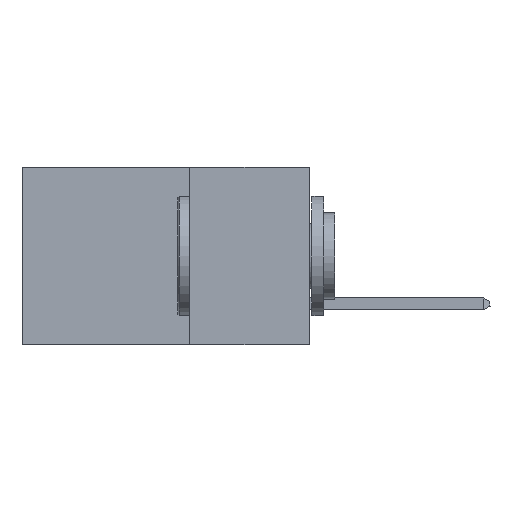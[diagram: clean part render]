
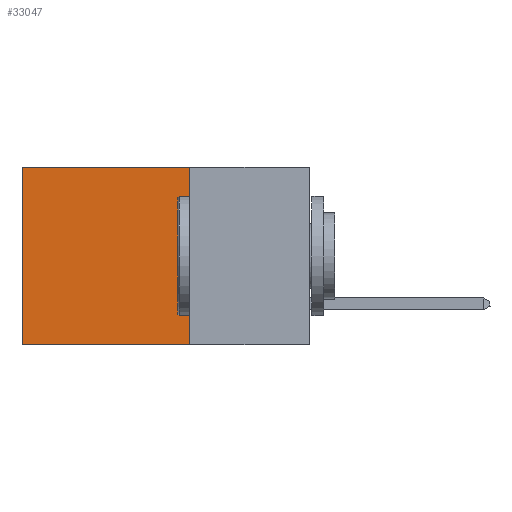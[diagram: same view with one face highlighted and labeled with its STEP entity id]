
A CAD part, left-side view. The second image highlights one B-rep face of the part: STEP entity #33047.
In plain terms, the highlighted planar face has unit normal (-1, 0, 0).
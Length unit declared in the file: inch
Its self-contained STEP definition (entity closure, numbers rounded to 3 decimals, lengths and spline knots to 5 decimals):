
#314 = EDGE_LOOP ( 'NONE', ( #17329, #42814, #28331, #37899 ) ) ;
#383 = CARTESIAN_POINT ( 'NONE',  ( 0.2875, 0.6, 0. ) ) ;
#529 = DIRECTION ( 'NONE',  ( 0., 0., -1. ) ) ;
#649 = DIRECTION ( 'NONE',  ( 0., 1., 0. ) ) ;
#990 = EDGE_CURVE ( 'NONE', #27193, #34456, #35570, .T. ) ;
#1653 = VECTOR ( 'NONE', #649, 39.37008 ) ;
#2077 = LINE ( 'NONE', #28543, #31311 ) ;
#3581 = CARTESIAN_POINT ( 'NONE',  ( 0.2875, 0.25, 0. ) ) ;
#4102 = CARTESIAN_POINT ( 'NONE',  ( 0.2875, 0.6, 0. ) ) ;
#4254 = EDGE_CURVE ( 'NONE', #19023, #27193, #28763, .T. ) ;
#4801 = DIRECTION ( 'NONE',  ( 1., 0., 0. ) ) ;
#6359 = VECTOR ( 'NONE', #32481, 39.37008 ) ;
#13077 = DIRECTION ( 'NONE',  ( 0., 1., 0. ) ) ;
#17329 = ORIENTED_EDGE ( 'NONE', *, *, #990, .T. ) ;
#18029 = CARTESIAN_POINT ( 'NONE',  ( 0.2875, 0.25, 0. ) ) ;
#19023 = VERTEX_POINT ( 'NONE', #3581 ) ;
#20257 = EDGE_CURVE ( 'NONE', #20815, #34456, #2077, .T. ) ;
#20815 = VERTEX_POINT ( 'NONE', #23988 ) ;
#23988 = CARTESIAN_POINT ( 'NONE',  ( 0.2875, 0.25, -0.37 ) ) ;
#25125 = CARTESIAN_POINT ( 'NONE',  ( 0.2875, 0.25, 0. ) ) ;
#25459 = LINE ( 'NONE', #36368, #6359 ) ;
#26327 = CARTESIAN_POINT ( 'NONE',  ( 0.2875, 0.6, -0.37 ) ) ;
#26534 = VECTOR ( 'NONE', #529, 39.37008 ) ;
#27193 = VERTEX_POINT ( 'NONE', #4102 ) ;
#28331 = ORIENTED_EDGE ( 'NONE', *, *, #29042, .F. ) ;
#28543 = CARTESIAN_POINT ( 'NONE',  ( 0.2875, 0.25, -0.37 ) ) ;
#28763 = LINE ( 'NONE', #18029, #1653 ) ;
#28873 = PLANE ( 'NONE',  #33361 ) ;
#29042 = EDGE_CURVE ( 'NONE', #19023, #20815, #25459, .T. ) ;
#29161 = DIRECTION ( 'NONE',  ( 0., 0., -1. ) ) ;
#31311 = VECTOR ( 'NONE', #13077, 39.37008 ) ;
#32481 = DIRECTION ( 'NONE',  ( 0., 0., -1. ) ) ;
#33047 = ADVANCED_FACE ( 'NONE', ( #38387 ), #28873, .F. ) ;
#33361 = AXIS2_PLACEMENT_3D ( 'NONE', #25125, #4801, #29161 ) ;
#34456 = VERTEX_POINT ( 'NONE', #26327 ) ;
#35570 = LINE ( 'NONE', #383, #26534 ) ;
#36368 = CARTESIAN_POINT ( 'NONE',  ( 0.2875, 0.25, 0. ) ) ;
#37899 = ORIENTED_EDGE ( 'NONE', *, *, #4254, .T. ) ;
#38387 = FACE_OUTER_BOUND ( 'NONE', #314, .T. ) ;
#42814 = ORIENTED_EDGE ( 'NONE', *, *, #20257, .F. ) ;
